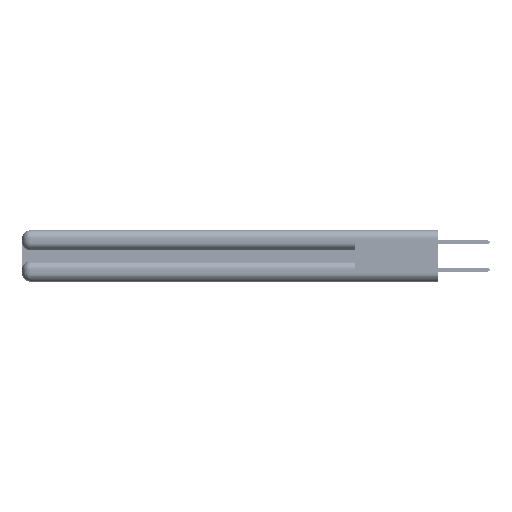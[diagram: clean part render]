
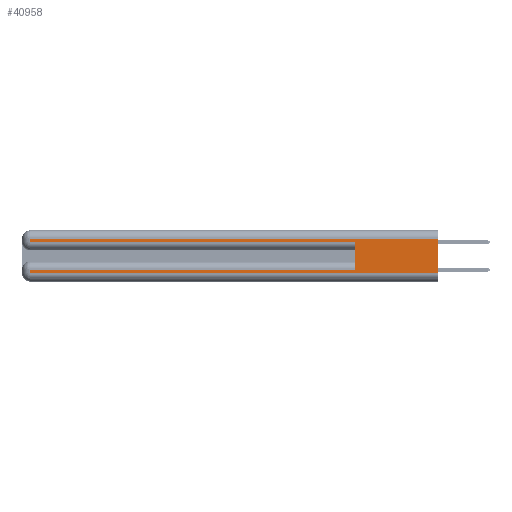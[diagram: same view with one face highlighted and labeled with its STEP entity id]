
A CAD part, left-side view. The second image highlights one B-rep face of the part: STEP entity #40958.
In plain terms, the highlighted planar face has unit normal (-1, 0, 0).
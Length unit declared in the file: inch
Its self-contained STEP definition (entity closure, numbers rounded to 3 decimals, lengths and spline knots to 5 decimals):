
#975 = VECTOR ( 'NONE', #19709, 39.37008 ) ;
#1726 = VERTEX_POINT ( 'NONE', #9467 ) ;
#2121 = CARTESIAN_POINT ( 'NONE',  ( 0., 0., 0.06 ) ) ;
#2259 = CARTESIAN_POINT ( 'NONE',  ( 0., 0., 0.06 ) ) ;
#2280 = FACE_OUTER_BOUND ( 'NONE', #4307, .T. ) ;
#2728 = LINE ( 'NONE', #14955, #47707 ) ;
#3888 = DIRECTION ( 'NONE',  ( 0., 1., 0. ) ) ;
#4307 = EDGE_LOOP ( 'NONE', ( #55130, #46864, #9914, #28688, #30361, #5787, #19186, #40294 ) ) ;
#4760 = EDGE_CURVE ( 'NONE', #29590, #7817, #49683, .T. ) ;
#5787 = ORIENTED_EDGE ( 'NONE', *, *, #55892, .T. ) ;
#6570 = AXIS2_PLACEMENT_3D ( 'NONE', #12861, #52246, #26258 ) ;
#7817 = VERTEX_POINT ( 'NONE', #33366 ) ;
#9467 = CARTESIAN_POINT ( 'NONE',  ( 0., 2.94, 0.06 ) ) ;
#9914 = ORIENTED_EDGE ( 'NONE', *, *, #51487, .T. ) ;
#10240 = CARTESIAN_POINT ( 'NONE',  ( 0., 2.94, 0.085 ) ) ;
#10309 = EDGE_CURVE ( 'NONE', #14660, #15882, #2728, .T. ) ;
#11366 = VECTOR ( 'NONE', #37103, 39.37008 ) ;
#12861 = CARTESIAN_POINT ( 'NONE',  ( 0., 0., 0.37 ) ) ;
#13052 = PLANE ( 'NONE',  #6570 ) ;
#13719 = VECTOR ( 'NONE', #20837, 39.37008 ) ;
#14660 = VERTEX_POINT ( 'NONE', #28513 ) ;
#14863 = CARTESIAN_POINT ( 'NONE',  ( 0., 2.94, 0.31 ) ) ;
#14955 = CARTESIAN_POINT ( 'NONE',  ( 0., 0., 0.37 ) ) ;
#15391 = CARTESIAN_POINT ( 'NONE',  ( 0., 2.94, 0.37 ) ) ;
#15406 = EDGE_CURVE ( 'NONE', #20573, #7817, #25369, .T. ) ;
#15882 = VERTEX_POINT ( 'NONE', #2259 ) ;
#17610 = CARTESIAN_POINT ( 'NONE',  ( 0., 0.6, 0.145 ) ) ;
#18073 = VECTOR ( 'NONE', #18470, 39.37008 ) ;
#18470 = DIRECTION ( 'NONE',  ( 0., 1., 0. ) ) ;
#19186 = ORIENTED_EDGE ( 'NONE', *, *, #29270, .T. ) ;
#19709 = DIRECTION ( 'NONE',  ( 0., -1., 0. ) ) ;
#20062 = VECTOR ( 'NONE', #3888, 39.37008 ) ;
#20573 = VERTEX_POINT ( 'NONE', #27197 ) ;
#20837 = DIRECTION ( 'NONE',  ( 0., -1., 0. ) ) ;
#23744 = DIRECTION ( 'NONE',  ( 0., 0., -1. ) ) ;
#23758 = DIRECTION ( 'NONE',  ( 0., 0., -1. ) ) ;
#25369 = LINE ( 'NONE', #46860, #13719 ) ;
#25430 = CARTESIAN_POINT ( 'NONE',  ( 0., 0.6, 0.085 ) ) ;
#26258 = DIRECTION ( 'NONE',  ( 0., 0., -1. ) ) ;
#27026 = LINE ( 'NONE', #45352, #37220 ) ;
#27197 = CARTESIAN_POINT ( 'NONE',  ( 0., 2.94, 0.285 ) ) ;
#28513 = CARTESIAN_POINT ( 'NONE',  ( 0., 0., 0.31 ) ) ;
#28688 = ORIENTED_EDGE ( 'NONE', *, *, #15406, .T. ) ;
#29270 = EDGE_CURVE ( 'NONE', #51353, #1726, #27026, .T. ) ;
#29590 = VERTEX_POINT ( 'NONE', #25430 ) ;
#29630 = LINE ( 'NONE', #35769, #18073 ) ;
#30361 = ORIENTED_EDGE ( 'NONE', *, *, #4760, .F. ) ;
#33366 = CARTESIAN_POINT ( 'NONE',  ( 0., 0.6, 0.285 ) ) ;
#34583 = LINE ( 'NONE', #15391, #11366 ) ;
#35769 = CARTESIAN_POINT ( 'NONE',  ( 0., 0., 0.31 ) ) ;
#35792 = LINE ( 'NONE', #2121, #975 ) ;
#36180 = EDGE_CURVE ( 'NONE', #1726, #15882, #35792, .T. ) ;
#37103 = DIRECTION ( 'NONE',  ( 0., 0., -1. ) ) ;
#37220 = VECTOR ( 'NONE', #23744, 39.37008 ) ;
#40294 = ORIENTED_EDGE ( 'NONE', *, *, #36180, .T. ) ;
#40958 = ADVANCED_FACE ( 'NONE', ( #2280 ), #13052, .F. ) ;
#43152 = CARTESIAN_POINT ( 'NONE',  ( 0., 0., 0.085 ) ) ;
#43171 = EDGE_CURVE ( 'NONE', #14660, #49795, #29630, .T. ) ;
#43657 = DIRECTION ( 'NONE',  ( 0., 0., 1. ) ) ;
#45352 = CARTESIAN_POINT ( 'NONE',  ( 0., 2.94, 0.37 ) ) ;
#46860 = CARTESIAN_POINT ( 'NONE',  ( 0., 0., 0.285 ) ) ;
#46864 = ORIENTED_EDGE ( 'NONE', *, *, #43171, .T. ) ;
#47707 = VECTOR ( 'NONE', #23758, 39.37008 ) ;
#48312 = VECTOR ( 'NONE', #43657, 39.37008 ) ;
#49683 = LINE ( 'NONE', #17610, #48312 ) ;
#49795 = VERTEX_POINT ( 'NONE', #14863 ) ;
#51353 = VERTEX_POINT ( 'NONE', #10240 ) ;
#51487 = EDGE_CURVE ( 'NONE', #49795, #20573, #34583, .T. ) ;
#52246 = DIRECTION ( 'NONE',  ( 1., 0., 0. ) ) ;
#54741 = LINE ( 'NONE', #43152, #20062 ) ;
#55130 = ORIENTED_EDGE ( 'NONE', *, *, #10309, .F. ) ;
#55892 = EDGE_CURVE ( 'NONE', #29590, #51353, #54741, .T. ) ;
